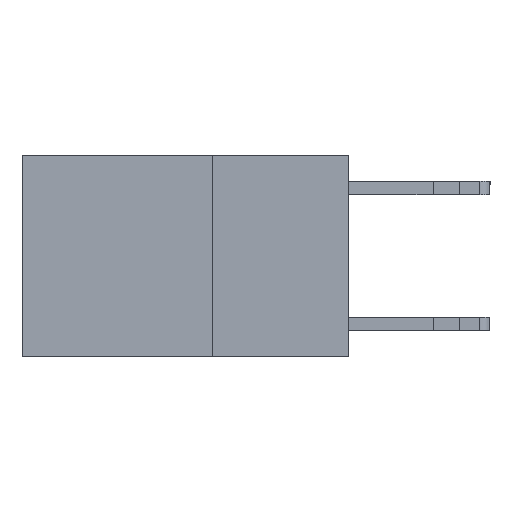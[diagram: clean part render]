
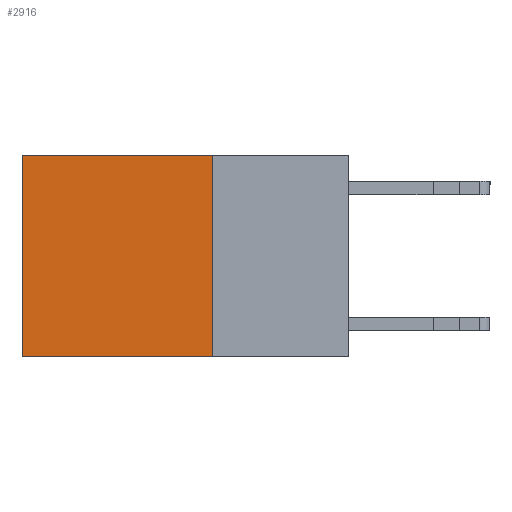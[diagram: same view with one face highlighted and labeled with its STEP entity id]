
A CAD part, left-side view. The second image highlights one B-rep face of the part: STEP entity #2916.
In plain terms, the highlighted planar face has unit normal (-1, 0, 0).
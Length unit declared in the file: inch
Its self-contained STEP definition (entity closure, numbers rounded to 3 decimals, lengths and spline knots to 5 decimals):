
#331 = VECTOR ( 'NONE', #6871, 39.37008 ) ;
#675 = CARTESIAN_POINT ( 'NONE',  ( 0.2625, 0.25, -0.37 ) ) ;
#996 = VERTEX_POINT ( 'NONE', #675 ) ;
#1137 = EDGE_LOOP ( 'NONE', ( #3225, #3515, #17543, #9608 ) ) ;
#1445 = LINE ( 'NONE', #5679, #13918 ) ;
#1859 = DIRECTION ( 'NONE',  ( 0., 1., 0. ) ) ;
#1936 = DIRECTION ( 'NONE',  ( 1., 0., 0. ) ) ;
#2916 = ADVANCED_FACE ( 'NONE', ( #16851 ), #14356, .F. ) ;
#3225 = ORIENTED_EDGE ( 'NONE', *, *, #12771, .T. ) ;
#3437 = LINE ( 'NONE', #7561, #14604 ) ;
#3515 = ORIENTED_EDGE ( 'NONE', *, *, #11277, .F. ) ;
#4150 = CARTESIAN_POINT ( 'NONE',  ( 0.2625, 0.6, 0. ) ) ;
#4843 = DIRECTION ( 'NONE',  ( 0., 0., -1. ) ) ;
#5508 = LINE ( 'NONE', #4150, #331 ) ;
#5679 = CARTESIAN_POINT ( 'NONE',  ( 0.2625, 0.25, 0. ) ) ;
#5900 = DIRECTION ( 'NONE',  ( 0., 0., -1. ) ) ;
#6871 = DIRECTION ( 'NONE',  ( 0., 0., -1. ) ) ;
#6941 = EDGE_CURVE ( 'NONE', #15704, #996, #1445, .T. ) ;
#7369 = VERTEX_POINT ( 'NONE', #16259 ) ;
#7561 = CARTESIAN_POINT ( 'NONE',  ( 0.2625, 0.25, -0.37 ) ) ;
#8653 = CARTESIAN_POINT ( 'NONE',  ( 0.2625, 0.25, 0. ) ) ;
#8977 = EDGE_CURVE ( 'NONE', #15704, #16981, #10456, .T. ) ;
#9608 = ORIENTED_EDGE ( 'NONE', *, *, #8977, .T. ) ;
#10456 = LINE ( 'NONE', #8653, #17127 ) ;
#11277 = EDGE_CURVE ( 'NONE', #996, #7369, #3437, .T. ) ;
#11531 = AXIS2_PLACEMENT_3D ( 'NONE', #14193, #1936, #5900 ) ;
#12771 = EDGE_CURVE ( 'NONE', #16981, #7369, #5508, .T. ) ;
#12825 = CARTESIAN_POINT ( 'NONE',  ( 0.2625, 0.25, 0. ) ) ;
#13918 = VECTOR ( 'NONE', #4843, 39.37008 ) ;
#14193 = CARTESIAN_POINT ( 'NONE',  ( 0.2625, 0.25, 0. ) ) ;
#14356 = PLANE ( 'NONE',  #11531 ) ;
#14604 = VECTOR ( 'NONE', #17096, 39.37008 ) ;
#14725 = CARTESIAN_POINT ( 'NONE',  ( 0.2625, 0.6, 0. ) ) ;
#15704 = VERTEX_POINT ( 'NONE', #12825 ) ;
#16259 = CARTESIAN_POINT ( 'NONE',  ( 0.2625, 0.6, -0.37 ) ) ;
#16851 = FACE_OUTER_BOUND ( 'NONE', #1137, .T. ) ;
#16981 = VERTEX_POINT ( 'NONE', #14725 ) ;
#17096 = DIRECTION ( 'NONE',  ( 0., 1., 0. ) ) ;
#17127 = VECTOR ( 'NONE', #1859, 39.37008 ) ;
#17543 = ORIENTED_EDGE ( 'NONE', *, *, #6941, .F. ) ;
